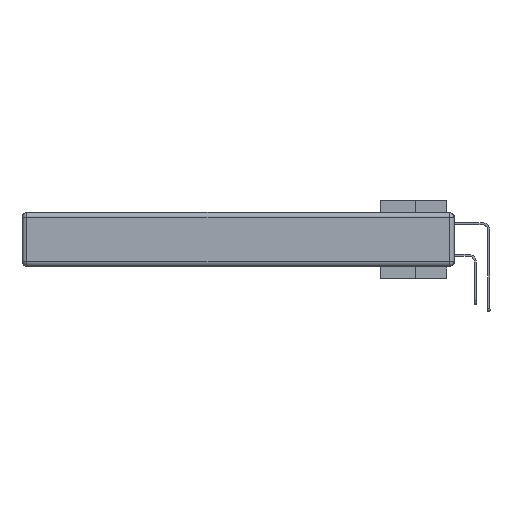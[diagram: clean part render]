
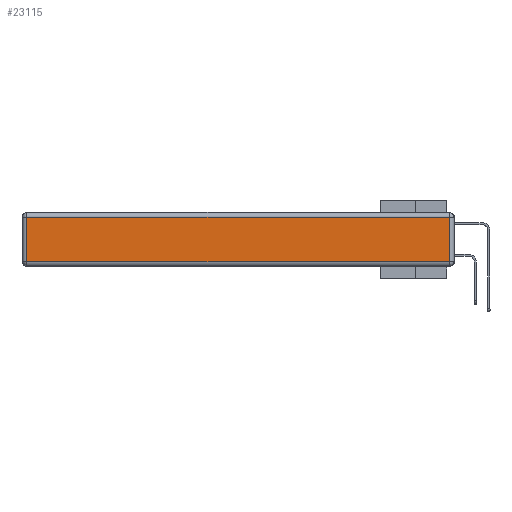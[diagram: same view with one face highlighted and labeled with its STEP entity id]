
A CAD part, left-side view. The second image highlights one B-rep face of the part: STEP entity #23115.
In plain terms, the highlighted planar face has unit normal (-1, 0, 0).
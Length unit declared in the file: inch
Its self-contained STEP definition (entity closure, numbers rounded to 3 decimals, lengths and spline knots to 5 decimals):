
#1509 = VERTEX_POINT ( 'NONE', #15249 ) ;
#3648 = DIRECTION ( 'NONE',  ( 0., 0., 1. ) ) ;
#3760 = CARTESIAN_POINT ( 'NONE',  ( 0., 2.75, -0.03 ) ) ;
#4121 = ORIENTED_EDGE ( 'NONE', *, *, #10814, .T. ) ;
#4200 = VERTEX_POINT ( 'NONE', #20381 ) ;
#4225 = LINE ( 'NONE', #30615, #10785 ) ;
#4239 = LINE ( 'NONE', #3760, #26955 ) ;
#5760 = PLANE ( 'NONE',  #22673 ) ;
#5940 = CARTESIAN_POINT ( 'NONE',  ( 0., 0., -0.313 ) ) ;
#6075 = FACE_OUTER_BOUND ( 'NONE', #27412, .T. ) ;
#6281 = VECTOR ( 'NONE', #15712, 39.37008 ) ;
#6790 = DIRECTION ( 'NONE',  ( 0., 0., 1. ) ) ;
#7240 = EDGE_CURVE ( 'NONE', #4200, #9866, #18090, .T. ) ;
#7263 = CARTESIAN_POINT ( 'NONE',  ( 0., 0.03, -0.313 ) ) ;
#8236 = EDGE_CURVE ( 'NONE', #9866, #1509, #4225, .T. ) ;
#8471 = DIRECTION ( 'NONE',  ( -1., 0., 0. ) ) ;
#9428 = CARTESIAN_POINT ( 'NONE',  ( 0., 2.72, -0.343 ) ) ;
#9866 = VERTEX_POINT ( 'NONE', #7263 ) ;
#10785 = VECTOR ( 'NONE', #6790, 39.37008 ) ;
#10814 = EDGE_CURVE ( 'NONE', #14603, #4200, #11830, .T. ) ;
#10867 = CARTESIAN_POINT ( 'NONE',  ( 0., 0., -0.343 ) ) ;
#11830 = LINE ( 'NONE', #9428, #12157 ) ;
#12157 = VECTOR ( 'NONE', #16955, 39.37008 ) ;
#14603 = VERTEX_POINT ( 'NONE', #18983 ) ;
#15249 = CARTESIAN_POINT ( 'NONE',  ( 0., 0.03, -0.03 ) ) ;
#15712 = DIRECTION ( 'NONE',  ( 0., -1., 0. ) ) ;
#15887 = ORIENTED_EDGE ( 'NONE', *, *, #8236, .T. ) ;
#16955 = DIRECTION ( 'NONE',  ( 0., 0., -1. ) ) ;
#17646 = EDGE_CURVE ( 'NONE', #1509, #14603, #4239, .T. ) ;
#18090 = LINE ( 'NONE', #5940, #6281 ) ;
#18191 = DIRECTION ( 'NONE',  ( 0., 1., 0. ) ) ;
#18983 = CARTESIAN_POINT ( 'NONE',  ( 0., 2.72, -0.03 ) ) ;
#20375 = ORIENTED_EDGE ( 'NONE', *, *, #7240, .T. ) ;
#20381 = CARTESIAN_POINT ( 'NONE',  ( 0., 2.72, -0.313 ) ) ;
#22673 = AXIS2_PLACEMENT_3D ( 'NONE', #10867, #8471, #3648 ) ;
#23115 = ADVANCED_FACE ( 'NONE', ( #6075 ), #5760, .T. ) ;
#25425 = ORIENTED_EDGE ( 'NONE', *, *, #17646, .T. ) ;
#26955 = VECTOR ( 'NONE', #18191, 39.37008 ) ;
#27412 = EDGE_LOOP ( 'NONE', ( #20375, #15887, #25425, #4121 ) ) ;
#30615 = CARTESIAN_POINT ( 'NONE',  ( 0., 0.03, -0.343 ) ) ;
